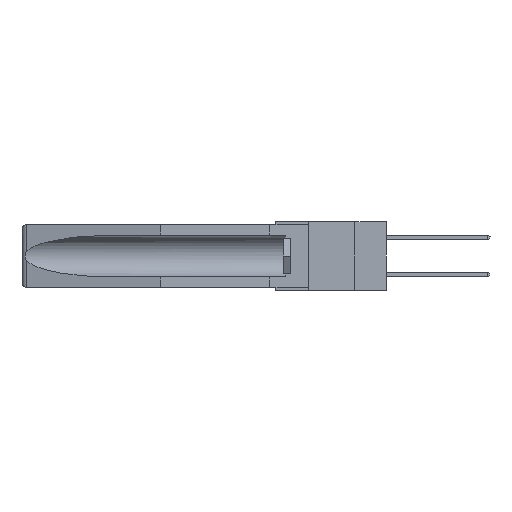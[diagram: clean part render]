
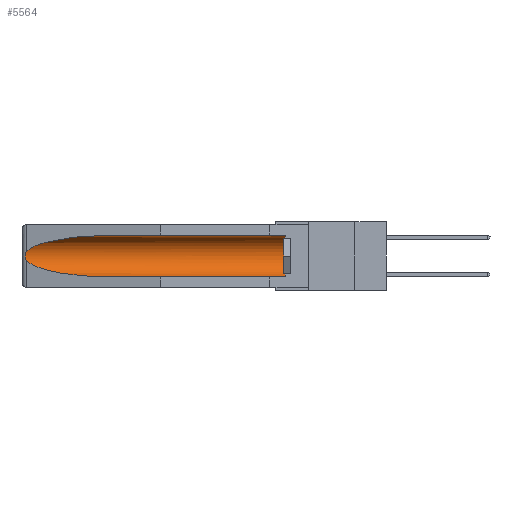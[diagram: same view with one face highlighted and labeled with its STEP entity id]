
A CAD part, left-side view. The second image highlights one B-rep face of the part: STEP entity #5564.
In plain terms, the highlighted cylindrical face has radius 2.857 mm (diameter 5.715 mm), a partial arc.
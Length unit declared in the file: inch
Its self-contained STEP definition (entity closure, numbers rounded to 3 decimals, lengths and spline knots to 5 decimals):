
#359 = EDGE_CURVE ( 'NONE', #701, #22185, #23969, .T. ) ;
#701 = VERTEX_POINT ( 'NONE', #25453 ) ;
#937 = CARTESIAN_POINT ( 'NONE',  ( 0.155, -0.30754, -0.284 ) ) ;
#1159 = DIRECTION ( 'NONE',  ( 0., 1., 0. ) ) ;
#1208 = DIRECTION ( 'NONE',  ( 0., 0., 1. ) ) ;
#2295 = CARTESIAN_POINT ( 'NONE',  ( 0.155, 1.07973, -0.059 ) ) ;
#2619 =( BOUNDED_CURVE ( )  B_SPLINE_CURVE ( 3, ( #24757, #4939, #22698, #12945 ),
 .UNSPECIFIED., .F., .F. ) 
 B_SPLINE_CURVE_WITH_KNOTS ( ( 4, 4 ),
 ( 0.1948, 1.5708 ),
 .UNSPECIFIED. ) 
 CURVE ( )  GEOMETRIC_REPRESENTATION_ITEM ( )  RATIONAL_B_SPLINE_CURVE ( ( 1., 0.848, 0.848, 1. ) ) 
 REPRESENTATION_ITEM ( '' )  );
#3586 = VERTEX_POINT ( 'NONE', #13965 ) ;
#3780 = VECTOR ( 'NONE', #22374, 39.37008 ) ;
#3842 = VERTEX_POINT ( 'NONE', #16764 ) ;
#4364 = EDGE_LOOP ( 'NONE', ( #10327, #22343, #20944, #17897, #18771, #16097 ) ) ;
#4788 = CARTESIAN_POINT ( 'NONE',  ( 0.26597, 1.5296, -0.19026 ) ) ;
#4939 = CARTESIAN_POINT ( 'NONE',  ( 0.25451, 1.48313, -0.24835 ) ) ;
#5564 = ADVANCED_FACE ( 'NONE', ( #13240 ), #25270, .F. ) ;
#6215 = CARTESIAN_POINT ( 'NONE',  ( 0.155, -0.30754, -0.1715 ) ) ;
#6395 = CARTESIAN_POINT ( 'NONE',  ( 0.26654, 1.53092, -0.15636 ) ) ;
#6481 = CARTESIAN_POINT ( 'NONE',  ( 0.2675, 1.53308, -0.17534 ) ) ;
#7739 = LINE ( 'NONE', #937, #3780 ) ;
#8008 = DIRECTION ( 'NONE',  ( 0., 0., 1. ) ) ;
#8536 = CARTESIAN_POINT ( 'NONE',  ( 0.2675, 1.53308, -0.16763 ) ) ;
#8543 = CARTESIAN_POINT ( 'NONE',  ( 0.21114, 1.30732, -0.059 ) ) ;
#8822 = CARTESIAN_POINT ( 'NONE',  ( 0.155, 0.126, -0.1715 ) ) ;
#9579 = EDGE_CURVE ( 'NONE', #22828, #23805, #2619, .T. ) ;
#10276 = CARTESIAN_POINT ( 'NONE',  ( 0.26537, 1.52718, -0.14972 ) ) ;
#10327 = ORIENTED_EDGE ( 'NONE', *, *, #15357, .T. ) ;
#10444 = CARTESIAN_POINT ( 'NONE',  ( 0.2673, 1.5327, -0.16383 ) ) ;
#11185 = CARTESIAN_POINT ( 'NONE',  ( 0.155, -0.30754, -0.059 ) ) ;
#11431 = AXIS2_PLACEMENT_3D ( 'NONE', #6215, #14185, #8008 ) ;
#11989 = CARTESIAN_POINT ( 'NONE',  ( 0.155, 1.07973, -0.284 ) ) ;
#12191 = B_SPLINE_CURVE_WITH_KNOTS ( 'NONE', 3,
 ( #10276, #22286, #6395, #10444, #8536, #6481, #12596, #20278, #4788, #14388 ),
 .UNSPECIFIED., .F., .F.,
 ( 4, 2, 2, 2, 4 ),
 ( 0., 0.00029, 0.00058, 0.00087, 0.00117 ),
 .UNSPECIFIED. ) ;
#12596 = CARTESIAN_POINT ( 'NONE',  ( 0.2673, 1.53269, -0.17917 ) ) ;
#12945 = CARTESIAN_POINT ( 'NONE',  ( 0.155, 1.07973, -0.284 ) ) ;
#13240 = FACE_OUTER_BOUND ( 'NONE', #4364, .T. ) ;
#13965 = CARTESIAN_POINT ( 'NONE',  ( 0.155, 0.126, -0.284 ) ) ;
#14185 = DIRECTION ( 'NONE',  ( 0., 1., 0. ) ) ;
#14224 = EDGE_CURVE ( 'NONE', #3842, #22828, #12191, .T. ) ;
#14388 = CARTESIAN_POINT ( 'NONE',  ( 0.26537, 1.52718, -0.19328 ) ) ;
#14416 = CARTESIAN_POINT ( 'NONE',  ( 0.155, 1.07973, -0.059 ) ) ;
#15357 = EDGE_CURVE ( 'NONE', #22185, #3842, #25187, .T. ) ;
#16095 = CARTESIAN_POINT ( 'NONE',  ( 0.26537, 1.52718, -0.14972 ) ) ;
#16097 = ORIENTED_EDGE ( 'NONE', *, *, #359, .T. ) ;
#16764 = CARTESIAN_POINT ( 'NONE',  ( 0.26537, 1.52718, -0.14972 ) ) ;
#16815 = DIRECTION ( 'NONE',  ( 0., -1., 0. ) ) ;
#17897 = ORIENTED_EDGE ( 'NONE', *, *, #23541, .F. ) ;
#17972 = AXIS2_PLACEMENT_3D ( 'NONE', #8822, #16815, #1208 ) ;
#18161 = VECTOR ( 'NONE', #1159, 39.37008 ) ;
#18339 = CIRCLE ( 'NONE', #17972, 0.1125 ) ;
#18771 = ORIENTED_EDGE ( 'NONE', *, *, #22298, .T. ) ;
#20116 = CARTESIAN_POINT ( 'NONE',  ( 0.25451, 1.48313, -0.09465 ) ) ;
#20176 = CARTESIAN_POINT ( 'NONE',  ( 0.26537, 1.52718, -0.19328 ) ) ;
#20278 = CARTESIAN_POINT ( 'NONE',  ( 0.26655, 1.53094, -0.18657 ) ) ;
#20944 = ORIENTED_EDGE ( 'NONE', *, *, #9579, .T. ) ;
#22185 = VERTEX_POINT ( 'NONE', #14416 ) ;
#22286 = CARTESIAN_POINT ( 'NONE',  ( 0.26597, 1.52961, -0.15275 ) ) ;
#22298 = EDGE_CURVE ( 'NONE', #3586, #701, #18339, .T. ) ;
#22343 = ORIENTED_EDGE ( 'NONE', *, *, #14224, .T. ) ;
#22374 = DIRECTION ( 'NONE',  ( 0., 1., 0. ) ) ;
#22698 = CARTESIAN_POINT ( 'NONE',  ( 0.21114, 1.30732, -0.284 ) ) ;
#22828 = VERTEX_POINT ( 'NONE', #20176 ) ;
#23541 = EDGE_CURVE ( 'NONE', #3586, #23805, #7739, .T. ) ;
#23805 = VERTEX_POINT ( 'NONE', #11989 ) ;
#23969 = LINE ( 'NONE', #11185, #18161 ) ;
#24757 = CARTESIAN_POINT ( 'NONE',  ( 0.26537, 1.52718, -0.19328 ) ) ;
#25187 =( BOUNDED_CURVE ( )  B_SPLINE_CURVE ( 3, ( #2295, #8543, #20116, #16095 ),
 .UNSPECIFIED., .F., .F. ) 
 B_SPLINE_CURVE_WITH_KNOTS ( ( 4, 4 ),
 ( 4.71239, 6.08839 ),
 .UNSPECIFIED. ) 
 CURVE ( )  GEOMETRIC_REPRESENTATION_ITEM ( )  RATIONAL_B_SPLINE_CURVE ( ( 1., 0.848, 0.848, 1. ) ) 
 REPRESENTATION_ITEM ( '' )  );
#25270 = CYLINDRICAL_SURFACE ( 'NONE', #11431, 0.1125 ) ;
#25453 = CARTESIAN_POINT ( 'NONE',  ( 0.155, 0.126, -0.059 ) ) ;
